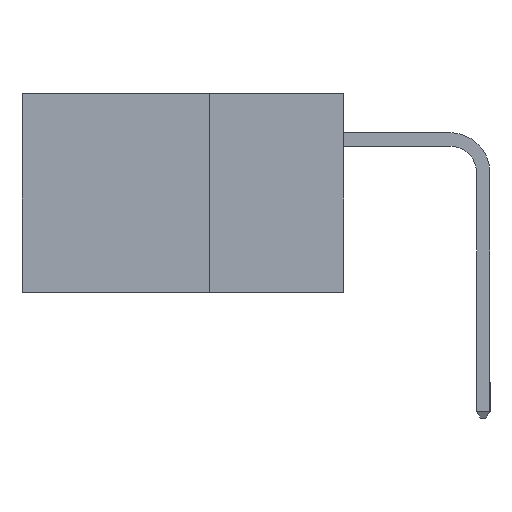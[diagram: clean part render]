
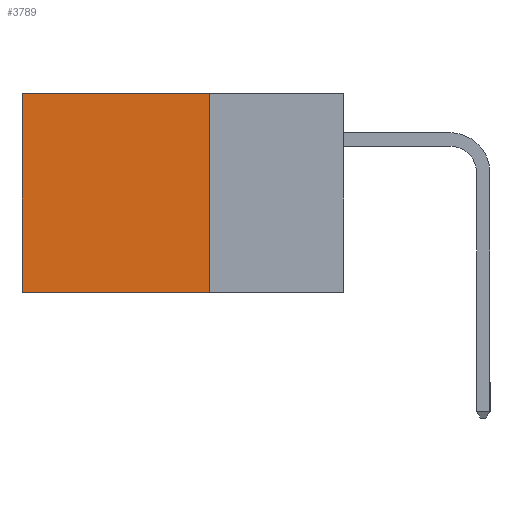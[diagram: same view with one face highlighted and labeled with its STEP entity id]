
A CAD part, left-side view. The second image highlights one B-rep face of the part: STEP entity #3789.
In plain terms, the highlighted planar face has unit normal (-1, 0, 0).
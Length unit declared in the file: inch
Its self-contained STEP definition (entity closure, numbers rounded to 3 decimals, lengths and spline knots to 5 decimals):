
#251 = CARTESIAN_POINT ( 'NONE',  ( 0.2615, 0.25, 0. ) ) ;
#2192 = DIRECTION ( 'NONE',  ( 1., 0., 0. ) ) ;
#2578 = LINE ( 'NONE', #7178, #7626 ) ;
#2636 = DIRECTION ( 'NONE',  ( 0., 0., -1. ) ) ;
#3081 = VECTOR ( 'NONE', #9388, 39.37008 ) ;
#3355 = ORIENTED_EDGE ( 'NONE', *, *, #4314, .T. ) ;
#3789 = ADVANCED_FACE ( 'NONE', ( #9591 ), #6911, .F. ) ;
#4314 = EDGE_CURVE ( 'NONE', #10754, #7019, #2578, .T. ) ;
#4917 = DIRECTION ( 'NONE',  ( 0., 1., 0. ) ) ;
#5368 = CARTESIAN_POINT ( 'NONE',  ( 0.2615, 0.25, 0. ) ) ;
#5494 = LINE ( 'NONE', #6429, #10450 ) ;
#5620 = AXIS2_PLACEMENT_3D ( 'NONE', #9528, #2192, #5979 ) ;
#5979 = DIRECTION ( 'NONE',  ( 0., 0., -1. ) ) ;
#6429 = CARTESIAN_POINT ( 'NONE',  ( 0.2615, 0.25, -0.37 ) ) ;
#6654 = CARTESIAN_POINT ( 'NONE',  ( 0.2615, 0.6, -0.37 ) ) ;
#6862 = EDGE_CURVE ( 'NONE', #7243, #7019, #9206, .T. ) ;
#6911 = PLANE ( 'NONE',  #5620 ) ;
#7019 = VERTEX_POINT ( 'NONE', #6654 ) ;
#7178 = CARTESIAN_POINT ( 'NONE',  ( 0.2615, 0.6, -0.37 ) ) ;
#7243 = VERTEX_POINT ( 'NONE', #7248 ) ;
#7248 = CARTESIAN_POINT ( 'NONE',  ( 0.2615, 0.25, -0.37 ) ) ;
#7331 = CARTESIAN_POINT ( 'NONE',  ( 0.2615, 0.25, -0.37 ) ) ;
#7419 = DIRECTION ( 'NONE',  ( 0., 0., -1. ) ) ;
#7626 = VECTOR ( 'NONE', #2636, 39.37008 ) ;
#7802 = EDGE_CURVE ( 'NONE', #7807, #7243, #5494, .T. ) ;
#7807 = VERTEX_POINT ( 'NONE', #5368 ) ;
#8097 = ORIENTED_EDGE ( 'NONE', *, *, #7802, .F. ) ;
#8553 = EDGE_LOOP ( 'NONE', ( #3355, #11923, #8097, #10439 ) ) ;
#8771 = LINE ( 'NONE', #251, #9690 ) ;
#9206 = LINE ( 'NONE', #7331, #3081 ) ;
#9352 = CARTESIAN_POINT ( 'NONE',  ( 0.2615, 0.6, 0. ) ) ;
#9388 = DIRECTION ( 'NONE',  ( 0., 1., 0. ) ) ;
#9528 = CARTESIAN_POINT ( 'NONE',  ( 0.2615, 0.25, -0.37 ) ) ;
#9591 = FACE_OUTER_BOUND ( 'NONE', #8553, .T. ) ;
#9641 = EDGE_CURVE ( 'NONE', #7807, #10754, #8771, .T. ) ;
#9690 = VECTOR ( 'NONE', #4917, 39.37008 ) ;
#10439 = ORIENTED_EDGE ( 'NONE', *, *, #9641, .T. ) ;
#10450 = VECTOR ( 'NONE', #7419, 39.37008 ) ;
#10754 = VERTEX_POINT ( 'NONE', #9352 ) ;
#11923 = ORIENTED_EDGE ( 'NONE', *, *, #6862, .F. ) ;
